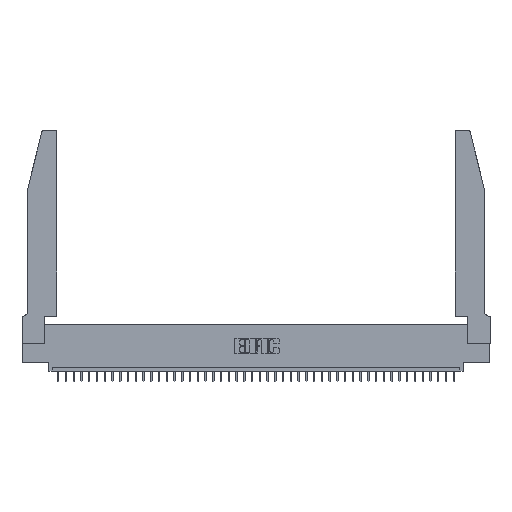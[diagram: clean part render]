
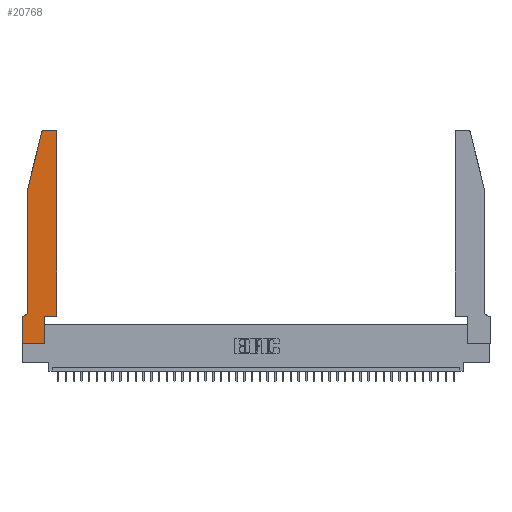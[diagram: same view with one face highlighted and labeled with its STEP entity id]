
A CAD part, top view. The second image highlights one B-rep face of the part: STEP entity #20768.
In plain terms, the highlighted planar face has unit normal (0, 0, 1).
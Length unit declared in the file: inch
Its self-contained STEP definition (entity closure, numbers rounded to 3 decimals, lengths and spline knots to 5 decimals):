
#11 = CIRCLE ( 'NONE', #3480, 0.03 ) ;
#217 = DIRECTION ( 'NONE',  ( 0., 0., 1. ) ) ;
#321 = EDGE_CURVE ( 'NONE', #6904, #16291, #35912, .T. ) ;
#1174 = VECTOR ( 'NONE', #22694, 39.37008 ) ;
#2598 = VERTEX_POINT ( 'NONE', #23394 ) ;
#2978 = PLANE ( 'NONE',  #13245 ) ;
#2985 = VECTOR ( 'NONE', #5529, 39.37008 ) ;
#3070 = EDGE_CURVE ( 'NONE', #8029, #38353, #11, .T. ) ;
#3266 = ORIENTED_EDGE ( 'NONE', *, *, #12594, .T. ) ;
#3480 = AXIS2_PLACEMENT_3D ( 'NONE', #13191, #217, #9939 ) ;
#3832 = LINE ( 'NONE', #10936, #29689 ) ;
#4314 = CARTESIAN_POINT ( 'NONE',  ( 0.4205, 2.75, 0.37 ) ) ;
#4586 = EDGE_CURVE ( 'NONE', #41872, #2598, #7698, .T. ) ;
#4668 = CARTESIAN_POINT ( 'NONE',  ( 0.4505, 0.35, 0.37 ) ) ;
#5529 = DIRECTION ( 'NONE',  ( -1., 0., 0. ) ) ;
#5630 = CARTESIAN_POINT ( 'NONE',  ( 0.0755, 2., 0.37 ) ) ;
#6262 = LINE ( 'NONE', #42599, #27640 ) ;
#6440 = EDGE_CURVE ( 'NONE', #6740, #8029, #12892, .T. ) ;
#6740 = VERTEX_POINT ( 'NONE', #4668 ) ;
#6904 = VERTEX_POINT ( 'NONE', #38830 ) ;
#7058 = FACE_OUTER_BOUND ( 'NONE', #11933, .T. ) ;
#7329 = VECTOR ( 'NONE', #29775, 39.37008 ) ;
#7698 = CIRCLE ( 'NONE', #38111, 0.07 ) ;
#8029 = VERTEX_POINT ( 'NONE', #10927 ) ;
#8122 = EDGE_CURVE ( 'NONE', #2598, #24942, #29282, .T. ) ;
#8390 = LINE ( 'NONE', #18746, #9425 ) ;
#9425 = VECTOR ( 'NONE', #15286, 39.37008 ) ;
#9595 = CARTESIAN_POINT ( 'NONE',  ( 0.0755, 0.35, 0.37 ) ) ;
#9770 = EDGE_CURVE ( 'NONE', #16291, #31884, #3832, .T. ) ;
#9939 = DIRECTION ( 'NONE',  ( 1., 0., 0. ) ) ;
#10015 = CARTESIAN_POINT ( 'NONE',  ( 0., 0.35, 0.37 ) ) ;
#10319 = DIRECTION ( 'NONE',  ( -1., 0., 0. ) ) ;
#10409 = ORIENTED_EDGE ( 'NONE', *, *, #8122, .T. ) ;
#10803 = LINE ( 'NONE', #20749, #40410 ) ;
#10927 = CARTESIAN_POINT ( 'NONE',  ( 0.4505, 2.72, 0.37 ) ) ;
#10936 = CARTESIAN_POINT ( 'NONE',  ( 0.0755, 2., 0.37 ) ) ;
#11933 = EDGE_LOOP ( 'NONE', ( #13071, #21029, #30836, #3266, #34005, #10409, #27450, #22399, #12001, #23392, #39200, #37233 ) ) ;
#12001 = ORIENTED_EDGE ( 'NONE', *, *, #22488, .T. ) ;
#12594 = EDGE_CURVE ( 'NONE', #31884, #41872, #28754, .T. ) ;
#12892 = LINE ( 'NONE', #38451, #38931 ) ;
#13071 = ORIENTED_EDGE ( 'NONE', *, *, #38478, .T. ) ;
#13191 = CARTESIAN_POINT ( 'NONE',  ( 0.4205, 2.72, 0.37 ) ) ;
#13245 = AXIS2_PLACEMENT_3D ( 'NONE', #30182, #33026, #22853 ) ;
#15286 = DIRECTION ( 'NONE',  ( -1., 0., 0. ) ) ;
#15410 = CARTESIAN_POINT ( 'NONE',  ( 0.0755, 0.42, 0.37 ) ) ;
#16291 = VERTEX_POINT ( 'NONE', #39894 ) ;
#16554 = CARTESIAN_POINT ( 'NONE',  ( 0.284, 2.72, 0.37 ) ) ;
#18746 = CARTESIAN_POINT ( 'NONE',  ( 0.2605, 2.75, 0.37 ) ) ;
#19098 = EDGE_CURVE ( 'NONE', #24942, #20069, #6262, .T. ) ;
#19209 = CARTESIAN_POINT ( 'NONE',  ( 0.0755, 2., 0.37 ) ) ;
#20069 = VERTEX_POINT ( 'NONE', #37292 ) ;
#20225 = VERTEX_POINT ( 'NONE', #35316 ) ;
#20307 = DIRECTION ( 'NONE',  ( 0., 1., 0. ) ) ;
#20444 = DIRECTION ( 'NONE',  ( 1., 0., 0. ) ) ;
#20749 = CARTESIAN_POINT ( 'NONE',  ( 0.4505, 0.35, 0.37 ) ) ;
#20768 = ADVANCED_FACE ( 'NONE', ( #7058 ), #2978, .T. ) ;
#21029 = ORIENTED_EDGE ( 'NONE', *, *, #321, .T. ) ;
#21251 = DIRECTION ( 'NONE',  ( 0., -1., 0. ) ) ;
#22399 = ORIENTED_EDGE ( 'NONE', *, *, #38030, .T. ) ;
#22488 = EDGE_CURVE ( 'NONE', #28537, #20225, #40024, .T. ) ;
#22694 = DIRECTION ( 'NONE',  ( 0., -1., 0. ) ) ;
#22853 = DIRECTION ( 'NONE',  ( 1., 0., 0. ) ) ;
#23392 = ORIENTED_EDGE ( 'NONE', *, *, #25480, .T. ) ;
#23394 = CARTESIAN_POINT ( 'NONE',  ( 0.0055, 0.35, 0.37 ) ) ;
#23929 = CARTESIAN_POINT ( 'NONE',  ( 0., 0., 0.37 ) ) ;
#24124 = DIRECTION ( 'NONE',  ( -0.239, -0.971, 0. ) ) ;
#24206 = DIRECTION ( 'NONE',  ( 1., 0., 0. ) ) ;
#24630 = CARTESIAN_POINT ( 'NONE',  ( 0.2865, 0., 0.37 ) ) ;
#24942 = VERTEX_POINT ( 'NONE', #10015 ) ;
#25480 = EDGE_CURVE ( 'NONE', #20225, #6740, #10803, .T. ) ;
#25651 = DIRECTION ( 'NONE',  ( 0., 1., 0. ) ) ;
#27048 = VECTOR ( 'NONE', #20307, 39.37008 ) ;
#27450 = ORIENTED_EDGE ( 'NONE', *, *, #19098, .T. ) ;
#27640 = VECTOR ( 'NONE', #21251, 39.37008 ) ;
#28537 = VERTEX_POINT ( 'NONE', #24630 ) ;
#28754 = LINE ( 'NONE', #5630, #1174 ) ;
#29282 = LINE ( 'NONE', #9595, #2985 ) ;
#29689 = VECTOR ( 'NONE', #24124, 39.37008 ) ;
#29751 = DIRECTION ( 'NONE',  ( 0., 0., 1. ) ) ;
#29775 = DIRECTION ( 'NONE',  ( 1., 0., 0. ) ) ;
#30182 = CARTESIAN_POINT ( 'NONE',  ( 0., 0.35, 0.37 ) ) ;
#30836 = ORIENTED_EDGE ( 'NONE', *, *, #9770, .T. ) ;
#31884 = VERTEX_POINT ( 'NONE', #19209 ) ;
#33026 = DIRECTION ( 'NONE',  ( 0., 0., 1. ) ) ;
#34005 = ORIENTED_EDGE ( 'NONE', *, *, #4586, .T. ) ;
#35316 = CARTESIAN_POINT ( 'NONE',  ( 0.2865, 0.35, 0.37 ) ) ;
#35875 = AXIS2_PLACEMENT_3D ( 'NONE', #16554, #29751, #20444 ) ;
#35912 = CIRCLE ( 'NONE', #35875, 0.03 ) ;
#37233 = ORIENTED_EDGE ( 'NONE', *, *, #3070, .T. ) ;
#37292 = CARTESIAN_POINT ( 'NONE',  ( 0., 0., 0.37 ) ) ;
#38030 = EDGE_CURVE ( 'NONE', #20069, #28537, #39763, .T. ) ;
#38111 = AXIS2_PLACEMENT_3D ( 'NONE', #39766, #42579, #10319 ) ;
#38353 = VERTEX_POINT ( 'NONE', #4314 ) ;
#38451 = CARTESIAN_POINT ( 'NONE',  ( 0.4505, 0.35, 0.37 ) ) ;
#38478 = EDGE_CURVE ( 'NONE', #38353, #6904, #8390, .T. ) ;
#38830 = CARTESIAN_POINT ( 'NONE',  ( 0.284, 2.75, 0.37 ) ) ;
#38931 = VECTOR ( 'NONE', #25651, 39.37008 ) ;
#39174 = CARTESIAN_POINT ( 'NONE',  ( 0.2865, 0.35, 0.37 ) ) ;
#39200 = ORIENTED_EDGE ( 'NONE', *, *, #6440, .T. ) ;
#39763 = LINE ( 'NONE', #23929, #7329 ) ;
#39766 = CARTESIAN_POINT ( 'NONE',  ( 0.0055, 0.42, 0.37 ) ) ;
#39894 = CARTESIAN_POINT ( 'NONE',  ( 0.25487, 2.72718, 0.37 ) ) ;
#40024 = LINE ( 'NONE', #39174, #27048 ) ;
#40410 = VECTOR ( 'NONE', #24206, 39.37008 ) ;
#41872 = VERTEX_POINT ( 'NONE', #15410 ) ;
#42579 = DIRECTION ( 'NONE',  ( 0., 0., -1. ) ) ;
#42599 = CARTESIAN_POINT ( 'NONE',  ( 0., 0., 0.37 ) ) ;
